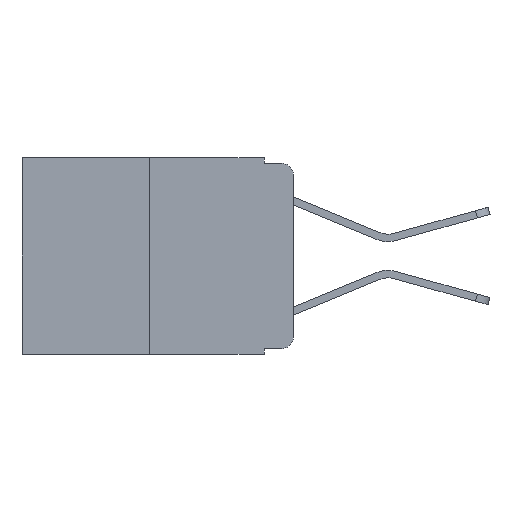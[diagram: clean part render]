
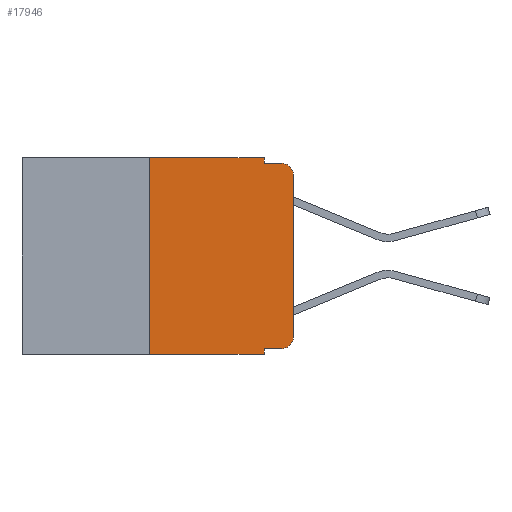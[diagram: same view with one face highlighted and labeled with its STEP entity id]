
A CAD part, left-side view. The second image highlights one B-rep face of the part: STEP entity #17946.
In plain terms, the highlighted planar face has unit normal (-1, 0, 0).
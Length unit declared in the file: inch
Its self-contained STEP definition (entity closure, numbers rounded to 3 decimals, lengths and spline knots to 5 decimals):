
#241 = DIRECTION ( 'NONE',  ( 0., 0., 1. ) ) ;
#658 = CARTESIAN_POINT ( 'NONE',  ( 0., 0.473, 0. ) ) ;
#750 = AXIS2_PLACEMENT_3D ( 'NONE', #11897, #2362, #13497 ) ;
#925 = CARTESIAN_POINT ( 'NONE',  ( 0., 0.473, 0. ) ) ;
#1285 = VECTOR ( 'NONE', #16421, 39.37008 ) ;
#1360 = VERTEX_POINT ( 'NONE', #16789 ) ;
#1449 = CARTESIAN_POINT ( 'NONE',  ( 0., 0., -0.03 ) ) ;
#1794 = LINE ( 'NONE', #14819, #1285 ) ;
#1797 = EDGE_CURVE ( 'NONE', #15579, #12352, #7792, .T. ) ;
#1980 = ORIENTED_EDGE ( 'NONE', *, *, #3158, .F. ) ;
#2337 = ORIENTED_EDGE ( 'NONE', *, *, #4826, .F. ) ;
#2362 = DIRECTION ( 'NONE',  ( -1., 0., 0. ) ) ;
#2376 = CARTESIAN_POINT ( 'NONE',  ( 0., 0.051, -0.01 ) ) ;
#2440 = CARTESIAN_POINT ( 'NONE',  ( 0., 0.02, -0.333 ) ) ;
#2615 = DIRECTION ( 'NONE',  ( 1., 0., 0. ) ) ;
#3064 = ORIENTED_EDGE ( 'NONE', *, *, #15324, .T. ) ;
#3158 = EDGE_CURVE ( 'NONE', #8055, #4260, #8702, .T. ) ;
#4260 = VERTEX_POINT ( 'NONE', #7363 ) ;
#4826 = EDGE_CURVE ( 'NONE', #15750, #12069, #19461, .T. ) ;
#4831 = VERTEX_POINT ( 'NONE', #18162 ) ;
#6523 = DIRECTION ( 'NONE',  ( -1., 0., 0. ) ) ;
#6693 = EDGE_CURVE ( 'NONE', #4831, #15676, #1794, .T. ) ;
#6747 = ORIENTED_EDGE ( 'NONE', *, *, #15261, .T. ) ;
#6919 = VECTOR ( 'NONE', #10344, 39.37008 ) ;
#6936 = AXIS2_PLACEMENT_3D ( 'NONE', #15976, #6523, #17530 ) ;
#7187 = VECTOR ( 'NONE', #15089, 39.37008 ) ;
#7330 = EDGE_CURVE ( 'NONE', #1360, #8055, #10571, .T. ) ;
#7363 = CARTESIAN_POINT ( 'NONE',  ( 0., 0.02, -0.01 ) ) ;
#7544 = DIRECTION ( 'NONE',  ( 0., -1., 0. ) ) ;
#7792 = LINE ( 'NONE', #13089, #11993 ) ;
#7961 = CIRCLE ( 'NONE', #750, 0.02 ) ;
#8055 = VERTEX_POINT ( 'NONE', #2376 ) ;
#8560 = CARTESIAN_POINT ( 'NONE',  ( 0., 0.25, -0.343 ) ) ;
#8702 = LINE ( 'NONE', #10619, #16635 ) ;
#8774 = EDGE_LOOP ( 'NONE', ( #13620, #14080, #1980, #20352, #19991, #9400, #3064, #2337, #6747, #10347 ) ) ;
#9059 = CIRCLE ( 'NONE', #6936, 0.02 ) ;
#9290 = DIRECTION ( 'NONE',  ( 0., -1., 0. ) ) ;
#9400 = ORIENTED_EDGE ( 'NONE', *, *, #1797, .F. ) ;
#9759 = AXIS2_PLACEMENT_3D ( 'NONE', #925, #2615, #13729 ) ;
#10099 = CARTESIAN_POINT ( 'NONE',  ( 0., 0.051, 0. ) ) ;
#10344 = DIRECTION ( 'NONE',  ( 0., 0., -1. ) ) ;
#10347 = ORIENTED_EDGE ( 'NONE', *, *, #14121, .T. ) ;
#10571 = LINE ( 'NONE', #10099, #14250 ) ;
#10583 = PLANE ( 'NONE',  #9759 ) ;
#10619 = CARTESIAN_POINT ( 'NONE',  ( 0., 0.051, -0.01 ) ) ;
#11403 = LINE ( 'NONE', #658, #7187 ) ;
#11606 = CARTESIAN_POINT ( 'NONE',  ( 0., 0.25, 0. ) ) ;
#11833 = EDGE_CURVE ( 'NONE', #15676, #4260, #7961, .T. ) ;
#11897 = CARTESIAN_POINT ( 'NONE',  ( 0., 0.02, -0.03 ) ) ;
#11993 = VECTOR ( 'NONE', #241, 39.37008 ) ;
#12069 = VERTEX_POINT ( 'NONE', #12444 ) ;
#12352 = VERTEX_POINT ( 'NONE', #11606 ) ;
#12444 = CARTESIAN_POINT ( 'NONE',  ( 0., 0.051, -0.343 ) ) ;
#13089 = CARTESIAN_POINT ( 'NONE',  ( 0., 0.25, 0. ) ) ;
#13251 = DIRECTION ( 'NONE',  ( 0., 0., -1. ) ) ;
#13497 = DIRECTION ( 'NONE',  ( 0., 0., -1. ) ) ;
#13620 = ORIENTED_EDGE ( 'NONE', *, *, #6693, .T. ) ;
#13729 = DIRECTION ( 'NONE',  ( 0., 0., -1. ) ) ;
#14080 = ORIENTED_EDGE ( 'NONE', *, *, #11833, .T. ) ;
#14121 = EDGE_CURVE ( 'NONE', #16632, #4831, #9059, .T. ) ;
#14250 = VECTOR ( 'NONE', #13251, 39.37008 ) ;
#14819 = CARTESIAN_POINT ( 'NONE',  ( 0., 0., 0. ) ) ;
#15089 = DIRECTION ( 'NONE',  ( 0., -1., 0. ) ) ;
#15103 = CARTESIAN_POINT ( 'NONE',  ( 0., 0.051, 0. ) ) ;
#15181 = VECTOR ( 'NONE', #15790, 39.37008 ) ;
#15261 = EDGE_CURVE ( 'NONE', #15750, #16632, #16657, .T. ) ;
#15324 = EDGE_CURVE ( 'NONE', #15579, #12069, #19311, .T. ) ;
#15579 = VERTEX_POINT ( 'NONE', #8560 ) ;
#15676 = VERTEX_POINT ( 'NONE', #1449 ) ;
#15750 = VERTEX_POINT ( 'NONE', #20548 ) ;
#15790 = DIRECTION ( 'NONE',  ( 0., -1., 0. ) ) ;
#15976 = CARTESIAN_POINT ( 'NONE',  ( 0., 0.02, -0.313 ) ) ;
#16172 = VECTOR ( 'NONE', #9290, 39.37008 ) ;
#16421 = DIRECTION ( 'NONE',  ( 0., 0., 1. ) ) ;
#16632 = VERTEX_POINT ( 'NONE', #2440 ) ;
#16635 = VECTOR ( 'NONE', #7544, 39.37008 ) ;
#16657 = LINE ( 'NONE', #17231, #16172 ) ;
#16789 = CARTESIAN_POINT ( 'NONE',  ( 0., 0.051, 0. ) ) ;
#17231 = CARTESIAN_POINT ( 'NONE',  ( 0., 0.051, -0.333 ) ) ;
#17240 = EDGE_CURVE ( 'NONE', #12352, #1360, #11403, .T. ) ;
#17530 = DIRECTION ( 'NONE',  ( 0., 0., -1. ) ) ;
#17946 = ADVANCED_FACE ( 'NONE', ( #18977 ), #10583, .F. ) ;
#18162 = CARTESIAN_POINT ( 'NONE',  ( 0., 0., -0.313 ) ) ;
#18977 = FACE_OUTER_BOUND ( 'NONE', #8774, .T. ) ;
#19311 = LINE ( 'NONE', #20386, #15181 ) ;
#19461 = LINE ( 'NONE', #15103, #6919 ) ;
#19991 = ORIENTED_EDGE ( 'NONE', *, *, #17240, .F. ) ;
#20352 = ORIENTED_EDGE ( 'NONE', *, *, #7330, .F. ) ;
#20386 = CARTESIAN_POINT ( 'NONE',  ( 0., 0.473, -0.343 ) ) ;
#20548 = CARTESIAN_POINT ( 'NONE',  ( 0., 0.051, -0.333 ) ) ;
